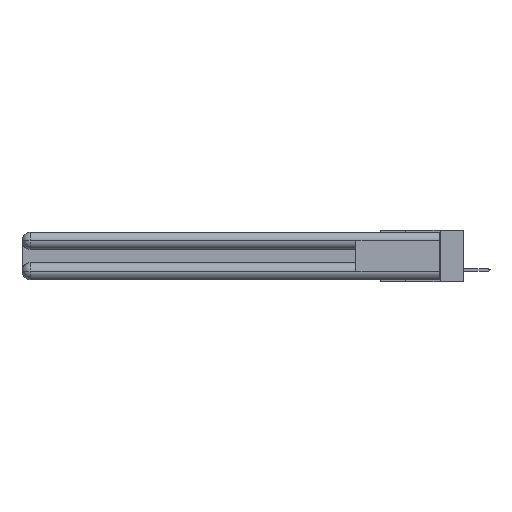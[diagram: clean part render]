
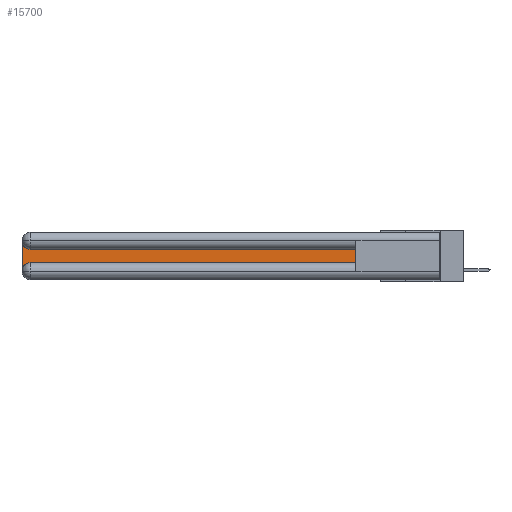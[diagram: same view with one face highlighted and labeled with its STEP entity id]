
A CAD part, left-side view. The second image highlights one B-rep face of the part: STEP entity #15700.
In plain terms, the highlighted planar face has unit normal (-1, 0, 0).
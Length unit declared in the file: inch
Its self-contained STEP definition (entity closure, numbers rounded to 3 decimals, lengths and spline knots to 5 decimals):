
#329 = DIRECTION ( 'NONE',  ( 1., 0., 0. ) ) ;
#2185 = CARTESIAN_POINT ( 'NONE',  ( 0.075, 3., -0.1225 ) ) ;
#2197 = AXIS2_PLACEMENT_3D ( 'NONE', #2445, #329, #17183 ) ;
#2445 = CARTESIAN_POINT ( 'NONE',  ( 0.075, 2.94, -0.2775 ) ) ;
#3202 = ORIENTED_EDGE ( 'NONE', *, *, #15663, .T. ) ;
#3770 = CARTESIAN_POINT ( 'NONE',  ( 0.075, 0.6, -0.2175 ) ) ;
#4332 = CARTESIAN_POINT ( 'NONE',  ( 0.075, 2.94, -0.1225 ) ) ;
#4843 = LINE ( 'NONE', #4948, #18708 ) ;
#4948 = CARTESIAN_POINT ( 'NONE',  ( 0.075, 0.6, -0.2175 ) ) ;
#5091 = DIRECTION ( 'NONE',  ( 0., 0., -1. ) ) ;
#5154 = VECTOR ( 'NONE', #18119, 39.37008 ) ;
#5820 = EDGE_LOOP ( 'NONE', ( #13004, #19702, #19158, #13481, #8427, #3202 ) ) ;
#6289 = DIRECTION ( 'NONE',  ( 0., 0., -1. ) ) ;
#6657 = VERTEX_POINT ( 'NONE', #21680 ) ;
#7497 = DIRECTION ( 'NONE',  ( 1., 0., 0. ) ) ;
#7871 = VERTEX_POINT ( 'NONE', #13244 ) ;
#8427 = ORIENTED_EDGE ( 'NONE', *, *, #11101, .T. ) ;
#8864 = CARTESIAN_POINT ( 'NONE',  ( 0.075, 2.94, -0.2175 ) ) ;
#9221 = EDGE_CURVE ( 'NONE', #19339, #6657, #27045, .T. ) ;
#9530 = VECTOR ( 'NONE', #24190, 39.37008 ) ;
#10348 = VERTEX_POINT ( 'NONE', #19242 ) ;
#10361 = PLANE ( 'NONE',  #21030 ) ;
#10774 = LINE ( 'NONE', #15986, #5154 ) ;
#11101 = EDGE_CURVE ( 'NONE', #14657, #10348, #24612, .T. ) ;
#13004 = ORIENTED_EDGE ( 'NONE', *, *, #15949, .T. ) ;
#13244 = CARTESIAN_POINT ( 'NONE',  ( 0.075, 0.6, -0.1225 ) ) ;
#13360 = VECTOR ( 'NONE', #25094, 39.37008 ) ;
#13481 = ORIENTED_EDGE ( 'NONE', *, *, #18812, .T. ) ;
#14466 = AXIS2_PLACEMENT_3D ( 'NONE', #21873, #7497, #5091 ) ;
#14615 = DIRECTION ( 'NONE',  ( 1., 0., 0. ) ) ;
#14657 = VERTEX_POINT ( 'NONE', #8864 ) ;
#14749 = FACE_OUTER_BOUND ( 'NONE', #5820, .T. ) ;
#15337 = VERTEX_POINT ( 'NONE', #4332 ) ;
#15663 = EDGE_CURVE ( 'NONE', #10348, #7871, #4843, .T. ) ;
#15686 = CARTESIAN_POINT ( 'NONE',  ( 0.075, 3., -0.2175 ) ) ;
#15700 = ADVANCED_FACE ( 'NONE', ( #14749 ), #10361, .F. ) ;
#15949 = EDGE_CURVE ( 'NONE', #7871, #15337, #10774, .T. ) ;
#15986 = CARTESIAN_POINT ( 'NONE',  ( 0.075, 0.6, -0.1225 ) ) ;
#16906 = CARTESIAN_POINT ( 'NONE',  ( 0.075, 3., -0.0625 ) ) ;
#17183 = DIRECTION ( 'NONE',  ( 0., 0., -1. ) ) ;
#18119 = DIRECTION ( 'NONE',  ( 0., 1., 0. ) ) ;
#18498 = CIRCLE ( 'NONE', #2197, 0.06 ) ;
#18708 = VECTOR ( 'NONE', #26745, 39.37008 ) ;
#18812 = EDGE_CURVE ( 'NONE', #6657, #14657, #18498, .T. ) ;
#19158 = ORIENTED_EDGE ( 'NONE', *, *, #9221, .T. ) ;
#19242 = CARTESIAN_POINT ( 'NONE',  ( 0.075, 0.6, -0.2175 ) ) ;
#19339 = VERTEX_POINT ( 'NONE', #16906 ) ;
#19702 = ORIENTED_EDGE ( 'NONE', *, *, #23891, .T. ) ;
#21030 = AXIS2_PLACEMENT_3D ( 'NONE', #2185, #14615, #6289 ) ;
#21680 = CARTESIAN_POINT ( 'NONE',  ( 0.075, 3., -0.2775 ) ) ;
#21873 = CARTESIAN_POINT ( 'NONE',  ( 0.075, 2.94, -0.0625 ) ) ;
#23891 = EDGE_CURVE ( 'NONE', #15337, #19339, #25309, .T. ) ;
#24190 = DIRECTION ( 'NONE',  ( 0., 0., -1. ) ) ;
#24612 = LINE ( 'NONE', #3770, #13360 ) ;
#25094 = DIRECTION ( 'NONE',  ( 0., -1., 0. ) ) ;
#25309 = CIRCLE ( 'NONE', #14466, 0.06 ) ;
#26745 = DIRECTION ( 'NONE',  ( 0., 0., 1. ) ) ;
#27045 = LINE ( 'NONE', #15686, #9530 ) ;
